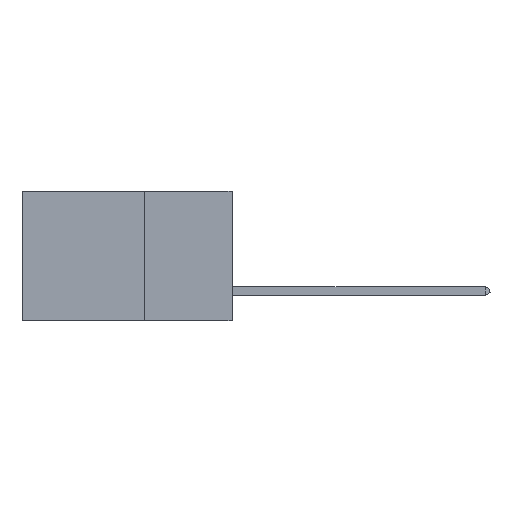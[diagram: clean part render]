
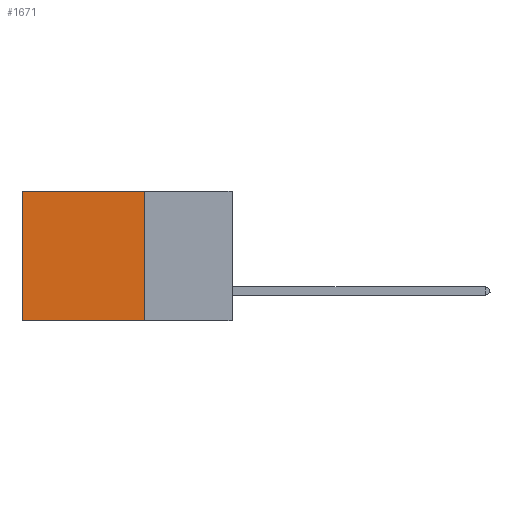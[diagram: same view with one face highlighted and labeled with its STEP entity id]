
A CAD part, left-side view. The second image highlights one B-rep face of the part: STEP entity #1671.
In plain terms, the highlighted planar face has unit normal (-1, 0, 0).
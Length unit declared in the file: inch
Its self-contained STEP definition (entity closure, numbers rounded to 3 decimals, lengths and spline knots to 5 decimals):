
#617 = CARTESIAN_POINT ( 'NONE',  ( 0.2875, 0.25, 0. ) ) ;
#834 = LINE ( 'NONE', #2088, #9241 ) ;
#1376 = DIRECTION ( 'NONE',  ( 0., 0., -1. ) ) ;
#1622 = DIRECTION ( 'NONE',  ( 0., 0., -1. ) ) ;
#1671 = ADVANCED_FACE ( 'NONE', ( #10224 ), #8325, .F. ) ;
#1813 = LINE ( 'NONE', #3931, #9356 ) ;
#1837 = VERTEX_POINT ( 'NONE', #12266 ) ;
#2088 = CARTESIAN_POINT ( 'NONE',  ( 0.2875, 0.25, -0.37 ) ) ;
#2458 = EDGE_LOOP ( 'NONE', ( #13730, #5441, #6432, #3795 ) ) ;
#2766 = DIRECTION ( 'NONE',  ( 0., 0., -1. ) ) ;
#2818 = DIRECTION ( 'NONE',  ( 1., 0., 0. ) ) ;
#2854 = CARTESIAN_POINT ( 'NONE',  ( 0.2875, 0.6, 0. ) ) ;
#2999 = CARTESIAN_POINT ( 'NONE',  ( 0.2875, 0.6, -0.37 ) ) ;
#3314 = CARTESIAN_POINT ( 'NONE',  ( 0.2875, 0.25, -0.37 ) ) ;
#3795 = ORIENTED_EDGE ( 'NONE', *, *, #6567, .T. ) ;
#3931 = CARTESIAN_POINT ( 'NONE',  ( 0.2875, 0.6, 0. ) ) ;
#4057 = VERTEX_POINT ( 'NONE', #2854 ) ;
#4147 = VECTOR ( 'NONE', #1376, 39.37008 ) ;
#4631 = AXIS2_PLACEMENT_3D ( 'NONE', #617, #2818, #2766 ) ;
#5391 = DIRECTION ( 'NONE',  ( 0., 1., 0. ) ) ;
#5441 = ORIENTED_EDGE ( 'NONE', *, *, #7665, .F. ) ;
#5963 = EDGE_CURVE ( 'NONE', #1837, #6529, #9770, .T. ) ;
#6432 = ORIENTED_EDGE ( 'NONE', *, *, #5963, .F. ) ;
#6529 = VERTEX_POINT ( 'NONE', #3314 ) ;
#6567 = EDGE_CURVE ( 'NONE', #1837, #4057, #11632, .T. ) ;
#6831 = CARTESIAN_POINT ( 'NONE',  ( 0.2875, 0.25, 0. ) ) ;
#7665 = EDGE_CURVE ( 'NONE', #6529, #9658, #834, .T. ) ;
#8233 = VECTOR ( 'NONE', #5391, 39.37008 ) ;
#8325 = PLANE ( 'NONE',  #4631 ) ;
#8546 = CARTESIAN_POINT ( 'NONE',  ( 0.2875, 0.25, 0. ) ) ;
#9241 = VECTOR ( 'NONE', #9663, 39.37008 ) ;
#9356 = VECTOR ( 'NONE', #1622, 39.37008 ) ;
#9658 = VERTEX_POINT ( 'NONE', #2999 ) ;
#9663 = DIRECTION ( 'NONE',  ( 0., 1., 0. ) ) ;
#9770 = LINE ( 'NONE', #6831, #4147 ) ;
#10224 = FACE_OUTER_BOUND ( 'NONE', #2458, .T. ) ;
#11632 = LINE ( 'NONE', #8546, #8233 ) ;
#12266 = CARTESIAN_POINT ( 'NONE',  ( 0.2875, 0.25, 0. ) ) ;
#13498 = EDGE_CURVE ( 'NONE', #4057, #9658, #1813, .T. ) ;
#13730 = ORIENTED_EDGE ( 'NONE', *, *, #13498, .T. ) ;
